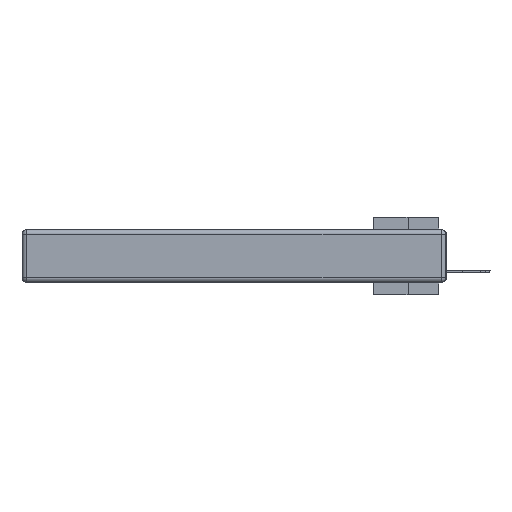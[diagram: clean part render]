
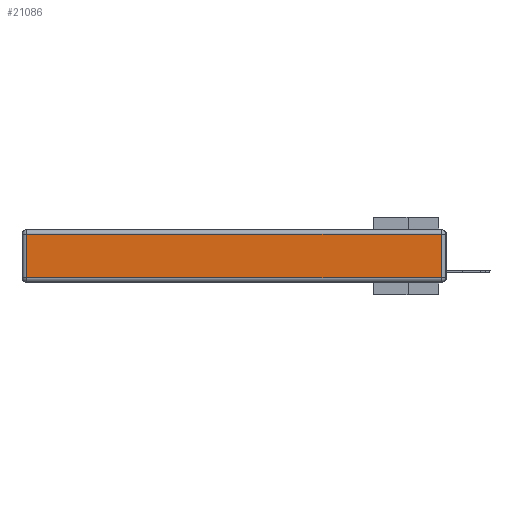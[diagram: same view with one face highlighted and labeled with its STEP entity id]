
A CAD part, left-side view. The second image highlights one B-rep face of the part: STEP entity #21086.
In plain terms, the highlighted planar face has unit normal (-1, 0, 0).
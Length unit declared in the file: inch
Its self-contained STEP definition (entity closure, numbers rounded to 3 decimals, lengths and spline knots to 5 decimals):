
#340 = ORIENTED_EDGE ( 'NONE', *, *, #19971, .T. ) ;
#2748 = CARTESIAN_POINT ( 'NONE',  ( 0., 0.03, -0.313 ) ) ;
#4696 = FACE_OUTER_BOUND ( 'NONE', #31574, .T. ) ;
#6307 = CARTESIAN_POINT ( 'NONE',  ( 0., 2.75, -0.03 ) ) ;
#6657 = CARTESIAN_POINT ( 'NONE',  ( 0., 0.03, -0.343 ) ) ;
#7724 = PLANE ( 'NONE',  #25007 ) ;
#7994 = DIRECTION ( 'NONE',  ( 0., 0., -1. ) ) ;
#9668 = CARTESIAN_POINT ( 'NONE',  ( 0., 0.03, -0.03 ) ) ;
#9696 = CARTESIAN_POINT ( 'NONE',  ( 0., 2.72, -0.313 ) ) ;
#9847 = LINE ( 'NONE', #6307, #32710 ) ;
#12508 = VECTOR ( 'NONE', #22810, 39.37008 ) ;
#12525 = DIRECTION ( 'NONE',  ( -1., 0., 0. ) ) ;
#14479 = VERTEX_POINT ( 'NONE', #9668 ) ;
#15472 = VERTEX_POINT ( 'NONE', #2748 ) ;
#18285 = VECTOR ( 'NONE', #23656, 39.37008 ) ;
#18339 = CARTESIAN_POINT ( 'NONE',  ( 0., 0., -0.313 ) ) ;
#18626 = CARTESIAN_POINT ( 'NONE',  ( 0., 2.72, -0.343 ) ) ;
#19153 = LINE ( 'NONE', #18626, #20396 ) ;
#19971 = EDGE_CURVE ( 'NONE', #15472, #14479, #25462, .T. ) ;
#20396 = VECTOR ( 'NONE', #7994, 39.37008 ) ;
#20648 = LINE ( 'NONE', #18339, #18285 ) ;
#20981 = VERTEX_POINT ( 'NONE', #9696 ) ;
#21086 = ADVANCED_FACE ( 'NONE', ( #4696 ), #7724, .T. ) ;
#22178 = ORIENTED_EDGE ( 'NONE', *, *, #24179, .T. ) ;
#22810 = DIRECTION ( 'NONE',  ( 0., 0., 1. ) ) ;
#23656 = DIRECTION ( 'NONE',  ( 0., -1., 0. ) ) ;
#24179 = EDGE_CURVE ( 'NONE', #20981, #15472, #20648, .T. ) ;
#25007 = AXIS2_PLACEMENT_3D ( 'NONE', #31674, #12525, #26000 ) ;
#25462 = LINE ( 'NONE', #6657, #12508 ) ;
#26000 = DIRECTION ( 'NONE',  ( 0., 0., 1. ) ) ;
#26350 = ORIENTED_EDGE ( 'NONE', *, *, #34135, .T. ) ;
#27300 = CARTESIAN_POINT ( 'NONE',  ( 0., 2.72, -0.03 ) ) ;
#29695 = VERTEX_POINT ( 'NONE', #27300 ) ;
#30617 = DIRECTION ( 'NONE',  ( 0., 1., 0. ) ) ;
#31474 = EDGE_CURVE ( 'NONE', #14479, #29695, #9847, .T. ) ;
#31574 = EDGE_LOOP ( 'NONE', ( #22178, #340, #33067, #26350 ) ) ;
#31674 = CARTESIAN_POINT ( 'NONE',  ( 0., 0., -0.343 ) ) ;
#32710 = VECTOR ( 'NONE', #30617, 39.37008 ) ;
#33067 = ORIENTED_EDGE ( 'NONE', *, *, #31474, .T. ) ;
#34135 = EDGE_CURVE ( 'NONE', #29695, #20981, #19153, .T. ) ;
